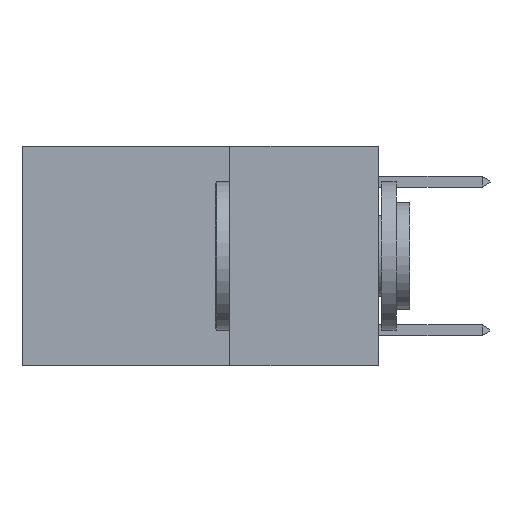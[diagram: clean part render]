
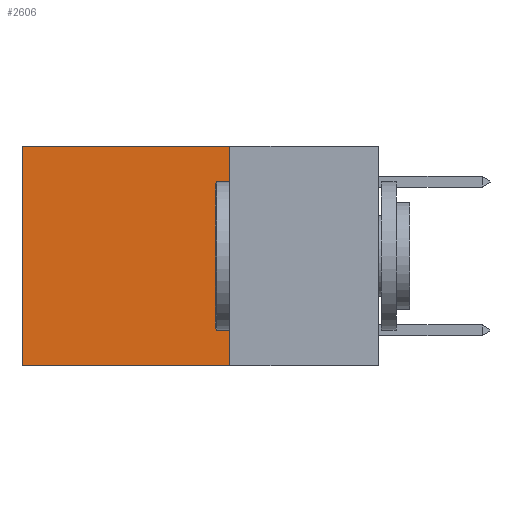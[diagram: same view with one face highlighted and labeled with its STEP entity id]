
A CAD part, left-side view. The second image highlights one B-rep face of the part: STEP entity #2606.
In plain terms, the highlighted planar face has unit normal (-1, 0, 0).
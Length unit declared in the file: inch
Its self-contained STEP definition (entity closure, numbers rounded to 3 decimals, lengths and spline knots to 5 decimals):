
#477 = LINE ( 'NONE', #9482, #13584 ) ;
#911 = VERTEX_POINT ( 'NONE', #8613 ) ;
#978 = DIRECTION ( 'NONE',  ( 0., 0., -1. ) ) ;
#1051 = DIRECTION ( 'NONE',  ( 1., 0., 0. ) ) ;
#2606 = ADVANCED_FACE ( 'NONE', ( #3853 ), #8792, .F. ) ;
#3059 = DIRECTION ( 'NONE',  ( 0., 1., 0. ) ) ;
#3206 = EDGE_LOOP ( 'NONE', ( #12308, #11557, #6141, #15679 ) ) ;
#3788 = EDGE_CURVE ( 'NONE', #7047, #911, #5026, .T. ) ;
#3853 = FACE_OUTER_BOUND ( 'NONE', #3206, .T. ) ;
#3903 = DIRECTION ( 'NONE',  ( 0., 0., -1. ) ) ;
#3969 = CARTESIAN_POINT ( 'NONE',  ( 0.2625, 0.25, 0. ) ) ;
#4276 = VECTOR ( 'NONE', #5264, 39.37008 ) ;
#4609 = CARTESIAN_POINT ( 'NONE',  ( 0.2625, 0.6, 0. ) ) ;
#4956 = LINE ( 'NONE', #9975, #15347 ) ;
#5026 = LINE ( 'NONE', #12785, #14670 ) ;
#5264 = DIRECTION ( 'NONE',  ( 0., 1., 0. ) ) ;
#6141 = ORIENTED_EDGE ( 'NONE', *, *, #3788, .F. ) ;
#7047 = VERTEX_POINT ( 'NONE', #13747 ) ;
#7352 = LINE ( 'NONE', #3969, #4276 ) ;
#8129 = EDGE_CURVE ( 'NONE', #9271, #9946, #4956, .T. ) ;
#8613 = CARTESIAN_POINT ( 'NONE',  ( 0.2625, 0.25, -0.37 ) ) ;
#8792 = PLANE ( 'NONE',  #14266 ) ;
#8894 = CARTESIAN_POINT ( 'NONE',  ( 0.2625, 0.6, -0.37 ) ) ;
#9271 = VERTEX_POINT ( 'NONE', #4609 ) ;
#9482 = CARTESIAN_POINT ( 'NONE',  ( 0.2625, 0.25, -0.37 ) ) ;
#9946 = VERTEX_POINT ( 'NONE', #8894 ) ;
#9975 = CARTESIAN_POINT ( 'NONE',  ( 0.2625, 0.6, 0. ) ) ;
#9995 = CARTESIAN_POINT ( 'NONE',  ( 0.2625, 0.25, 0. ) ) ;
#10055 = DIRECTION ( 'NONE',  ( 0., 0., -1. ) ) ;
#10985 = EDGE_CURVE ( 'NONE', #7047, #9271, #7352, .T. ) ;
#11557 = ORIENTED_EDGE ( 'NONE', *, *, #14182, .F. ) ;
#12308 = ORIENTED_EDGE ( 'NONE', *, *, #8129, .T. ) ;
#12785 = CARTESIAN_POINT ( 'NONE',  ( 0.2625, 0.25, 0. ) ) ;
#13584 = VECTOR ( 'NONE', #3059, 39.37008 ) ;
#13747 = CARTESIAN_POINT ( 'NONE',  ( 0.2625, 0.25, 0. ) ) ;
#14182 = EDGE_CURVE ( 'NONE', #911, #9946, #477, .T. ) ;
#14266 = AXIS2_PLACEMENT_3D ( 'NONE', #9995, #1051, #10055 ) ;
#14670 = VECTOR ( 'NONE', #3903, 39.37008 ) ;
#15347 = VECTOR ( 'NONE', #978, 39.37008 ) ;
#15679 = ORIENTED_EDGE ( 'NONE', *, *, #10985, .T. ) ;
